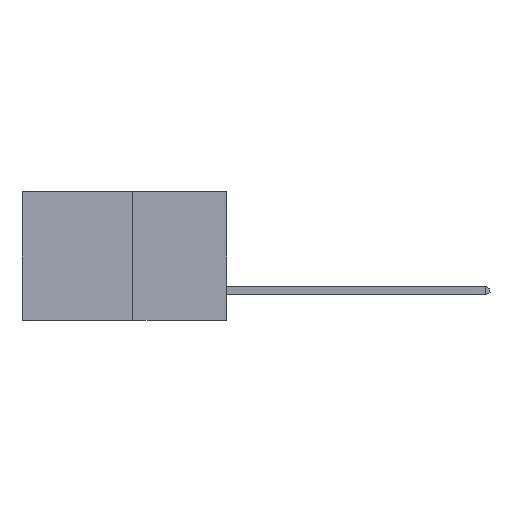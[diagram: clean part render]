
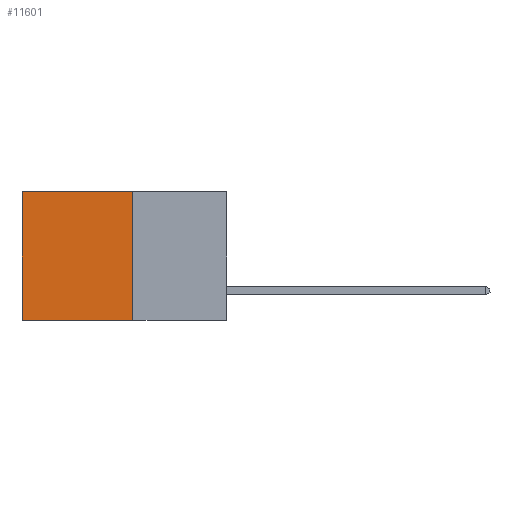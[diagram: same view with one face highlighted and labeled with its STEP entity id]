
A CAD part, left-side view. The second image highlights one B-rep face of the part: STEP entity #11601.
In plain terms, the highlighted planar face has unit normal (-1, 0, 0).
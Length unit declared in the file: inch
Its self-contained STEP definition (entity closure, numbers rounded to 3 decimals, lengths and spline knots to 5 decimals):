
#350 = CARTESIAN_POINT ( 'NONE',  ( 0.277, 0.27, -0.37 ) ) ;
#574 = EDGE_CURVE ( 'NONE', #3304, #5314, #4569, .T. ) ;
#1376 = DIRECTION ( 'NONE',  ( 0., 0., -1. ) ) ;
#1872 = EDGE_CURVE ( 'NONE', #2368, #3304, #5003, .T. ) ;
#1986 = LINE ( 'NONE', #3817, #4495 ) ;
#2368 = VERTEX_POINT ( 'NONE', #8154 ) ;
#3161 = DIRECTION ( 'NONE',  ( 0., 1., 0. ) ) ;
#3212 = CARTESIAN_POINT ( 'NONE',  ( 0.277, 0.27, -0.37 ) ) ;
#3304 = VERTEX_POINT ( 'NONE', #10892 ) ;
#3468 = EDGE_CURVE ( 'NONE', #2368, #7633, #1986, .T. ) ;
#3543 = CARTESIAN_POINT ( 'NONE',  ( 0.277, 0.27, -0.37 ) ) ;
#3675 = CARTESIAN_POINT ( 'NONE',  ( 0.277, 0.59, -0.37 ) ) ;
#3817 = CARTESIAN_POINT ( 'NONE',  ( 0.277, 0.27, -0.37 ) ) ;
#3948 = DIRECTION ( 'NONE',  ( 0., 0., -1. ) ) ;
#3967 = EDGE_CURVE ( 'NONE', #7633, #5314, #4952, .T. ) ;
#4495 = VECTOR ( 'NONE', #3948, 39.37008 ) ;
#4569 = LINE ( 'NONE', #6455, #6815 ) ;
#4604 = DIRECTION ( 'NONE',  ( 0., 1., 0. ) ) ;
#4952 = LINE ( 'NONE', #3212, #9429 ) ;
#5003 = LINE ( 'NONE', #5343, #8971 ) ;
#5314 = VERTEX_POINT ( 'NONE', #3675 ) ;
#5343 = CARTESIAN_POINT ( 'NONE',  ( 0.277, 0.27, 0. ) ) ;
#6455 = CARTESIAN_POINT ( 'NONE',  ( 0.277, 0.59, -0.37 ) ) ;
#6815 = VECTOR ( 'NONE', #11060, 39.37008 ) ;
#7368 = DIRECTION ( 'NONE',  ( 1., 0., 0. ) ) ;
#7633 = VERTEX_POINT ( 'NONE', #3543 ) ;
#8154 = CARTESIAN_POINT ( 'NONE',  ( 0.277, 0.27, 0. ) ) ;
#8212 = PLANE ( 'NONE',  #8342 ) ;
#8332 = ORIENTED_EDGE ( 'NONE', *, *, #574, .T. ) ;
#8342 = AXIS2_PLACEMENT_3D ( 'NONE', #350, #7368, #1376 ) ;
#8360 = ORIENTED_EDGE ( 'NONE', *, *, #1872, .T. ) ;
#8383 = ORIENTED_EDGE ( 'NONE', *, *, #3468, .F. ) ;
#8971 = VECTOR ( 'NONE', #4604, 39.37008 ) ;
#9429 = VECTOR ( 'NONE', #3161, 39.37008 ) ;
#9729 = EDGE_LOOP ( 'NONE', ( #8332, #11292, #8383, #8360 ) ) ;
#10892 = CARTESIAN_POINT ( 'NONE',  ( 0.277, 0.59, 0. ) ) ;
#11060 = DIRECTION ( 'NONE',  ( 0., 0., -1. ) ) ;
#11203 = FACE_OUTER_BOUND ( 'NONE', #9729, .T. ) ;
#11292 = ORIENTED_EDGE ( 'NONE', *, *, #3967, .F. ) ;
#11601 = ADVANCED_FACE ( 'NONE', ( #11203 ), #8212, .F. ) ;
